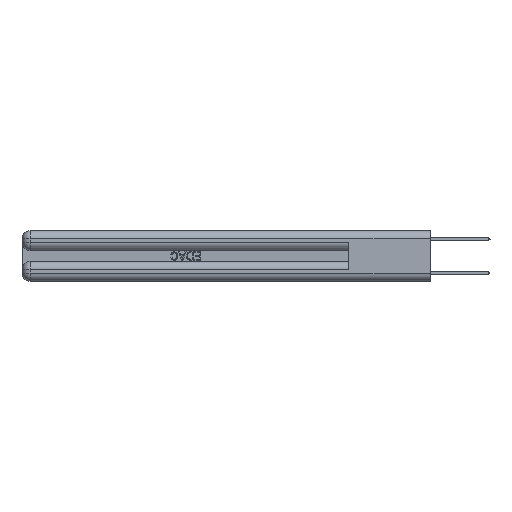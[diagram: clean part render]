
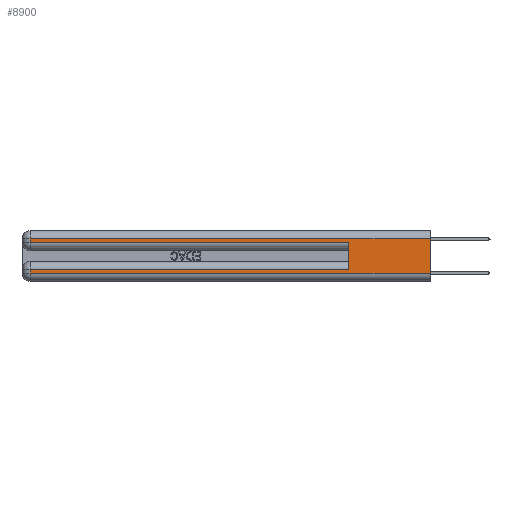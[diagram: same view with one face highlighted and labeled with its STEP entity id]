
A CAD part, left-side view. The second image highlights one B-rep face of the part: STEP entity #8900.
In plain terms, the highlighted planar face has unit normal (-1, 0, 0).
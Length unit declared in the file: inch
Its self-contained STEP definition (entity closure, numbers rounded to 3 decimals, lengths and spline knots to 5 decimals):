
#623 = CARTESIAN_POINT ( 'NONE',  ( 0., 0., 0.31 ) ) ;
#798 = VECTOR ( 'NONE', #12444, 39.37008 ) ;
#1790 = EDGE_CURVE ( 'NONE', #26164, #24683, #11118, .T. ) ;
#2555 = LINE ( 'NONE', #9027, #7145 ) ;
#2967 = DIRECTION ( 'NONE',  ( 0., 0., -1. ) ) ;
#3575 = LINE ( 'NONE', #28117, #26703 ) ;
#4040 = VECTOR ( 'NONE', #7746, 39.37008 ) ;
#4646 = CARTESIAN_POINT ( 'NONE',  ( 0., 0.6, 0.145 ) ) ;
#5130 = ORIENTED_EDGE ( 'NONE', *, *, #25326, .T. ) ;
#5353 = VECTOR ( 'NONE', #7558, 39.37008 ) ;
#5649 = CARTESIAN_POINT ( 'NONE',  ( 0., 2.94, 0.085 ) ) ;
#6205 = ORIENTED_EDGE ( 'NONE', *, *, #31006, .T. ) ;
#6625 = VERTEX_POINT ( 'NONE', #5649 ) ;
#7144 = DIRECTION ( 'NONE',  ( 0., 1., 0. ) ) ;
#7145 = VECTOR ( 'NONE', #11701, 39.37008 ) ;
#7558 = DIRECTION ( 'NONE',  ( 0., 0., 1. ) ) ;
#7746 = DIRECTION ( 'NONE',  ( 0., -1., 0. ) ) ;
#7767 = ORIENTED_EDGE ( 'NONE', *, *, #27927, .F. ) ;
#8213 = CARTESIAN_POINT ( 'NONE',  ( 0., 2.94, 0.37 ) ) ;
#8378 = CARTESIAN_POINT ( 'NONE',  ( 0., 0., 0.06 ) ) ;
#8900 = ADVANCED_FACE ( 'NONE', ( #31341 ), #32390, .F. ) ;
#9011 = VERTEX_POINT ( 'NONE', #27538 ) ;
#9027 = CARTESIAN_POINT ( 'NONE',  ( 0., 2.94, 0.37 ) ) ;
#9396 = LINE ( 'NONE', #8213, #31192 ) ;
#9757 = CARTESIAN_POINT ( 'NONE',  ( 0., 0., 0.37 ) ) ;
#10548 = CARTESIAN_POINT ( 'NONE',  ( 0., 0., 0.285 ) ) ;
#10793 = CARTESIAN_POINT ( 'NONE',  ( 0., 2.94, 0.285 ) ) ;
#11118 = LINE ( 'NONE', #10548, #4040 ) ;
#11310 = CARTESIAN_POINT ( 'NONE',  ( 0., 0.6, 0.285 ) ) ;
#11701 = DIRECTION ( 'NONE',  ( 0., 0., -1. ) ) ;
#12444 = DIRECTION ( 'NONE',  ( 0., 0., -1. ) ) ;
#12628 = EDGE_CURVE ( 'NONE', #20647, #6625, #21157, .T. ) ;
#13319 = CARTESIAN_POINT ( 'NONE',  ( 0., 0., 0.085 ) ) ;
#14786 = ORIENTED_EDGE ( 'NONE', *, *, #1790, .T. ) ;
#15686 = EDGE_CURVE ( 'NONE', #24755, #30839, #3575, .T. ) ;
#16612 = CARTESIAN_POINT ( 'NONE',  ( 0., 0., 0.37 ) ) ;
#17053 = VECTOR ( 'NONE', #18710, 39.37008 ) ;
#17367 = ORIENTED_EDGE ( 'NONE', *, *, #20152, .T. ) ;
#17937 = CARTESIAN_POINT ( 'NONE',  ( 0., 2.94, 0.31 ) ) ;
#17950 = EDGE_CURVE ( 'NONE', #24755, #9011, #29319, .T. ) ;
#17965 = VERTEX_POINT ( 'NONE', #20334 ) ;
#18710 = DIRECTION ( 'NONE',  ( 0., 1., 0. ) ) ;
#20152 = EDGE_CURVE ( 'NONE', #17965, #9011, #28753, .T. ) ;
#20334 = CARTESIAN_POINT ( 'NONE',  ( 0., 2.94, 0.06 ) ) ;
#20647 = VERTEX_POINT ( 'NONE', #21032 ) ;
#21032 = CARTESIAN_POINT ( 'NONE',  ( 0., 0.6, 0.085 ) ) ;
#21157 = LINE ( 'NONE', #13319, #17053 ) ;
#22609 = ORIENTED_EDGE ( 'NONE', *, *, #17950, .F. ) ;
#24459 = AXIS2_PLACEMENT_3D ( 'NONE', #16612, #29852, #24693 ) ;
#24683 = VERTEX_POINT ( 'NONE', #11310 ) ;
#24693 = DIRECTION ( 'NONE',  ( 0., 0., -1. ) ) ;
#24755 = VERTEX_POINT ( 'NONE', #623 ) ;
#25326 = EDGE_CURVE ( 'NONE', #6625, #17965, #2555, .T. ) ;
#26164 = VERTEX_POINT ( 'NONE', #10793 ) ;
#26703 = VECTOR ( 'NONE', #7144, 39.37008 ) ;
#26715 = DIRECTION ( 'NONE',  ( 0., -1., 0. ) ) ;
#27538 = CARTESIAN_POINT ( 'NONE',  ( 0., 0., 0.06 ) ) ;
#27927 = EDGE_CURVE ( 'NONE', #20647, #24683, #33415, .T. ) ;
#28117 = CARTESIAN_POINT ( 'NONE',  ( 0., 0., 0.31 ) ) ;
#28753 = LINE ( 'NONE', #8378, #33708 ) ;
#29319 = LINE ( 'NONE', #9757, #798 ) ;
#29431 = EDGE_LOOP ( 'NONE', ( #22609, #31410, #6205, #14786, #7767, #33967, #5130, #17367 ) ) ;
#29852 = DIRECTION ( 'NONE',  ( 1., 0., 0. ) ) ;
#30839 = VERTEX_POINT ( 'NONE', #17937 ) ;
#31006 = EDGE_CURVE ( 'NONE', #30839, #26164, #9396, .T. ) ;
#31192 = VECTOR ( 'NONE', #2967, 39.37008 ) ;
#31341 = FACE_OUTER_BOUND ( 'NONE', #29431, .T. ) ;
#31410 = ORIENTED_EDGE ( 'NONE', *, *, #15686, .T. ) ;
#32390 = PLANE ( 'NONE',  #24459 ) ;
#33415 = LINE ( 'NONE', #4646, #5353 ) ;
#33708 = VECTOR ( 'NONE', #26715, 39.37008 ) ;
#33967 = ORIENTED_EDGE ( 'NONE', *, *, #12628, .T. ) ;
